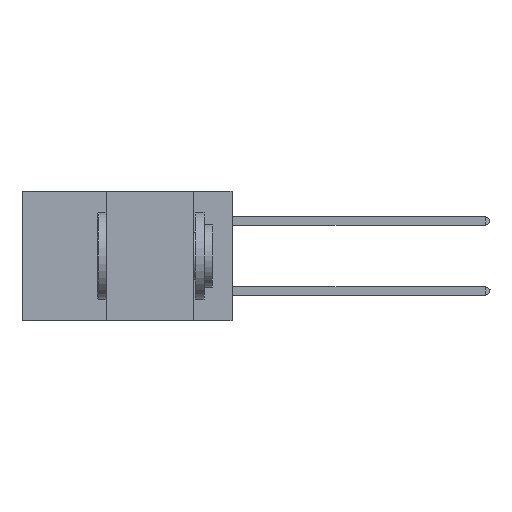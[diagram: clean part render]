
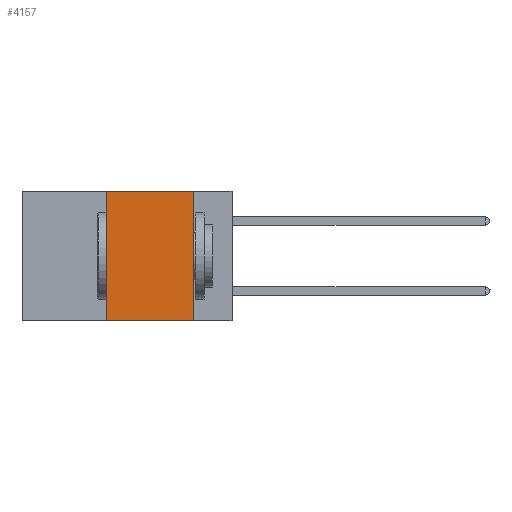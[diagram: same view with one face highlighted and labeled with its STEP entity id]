
A CAD part, left-side view. The second image highlights one B-rep face of the part: STEP entity #4157.
In plain terms, the highlighted planar face has unit normal (-1, 0, 0).
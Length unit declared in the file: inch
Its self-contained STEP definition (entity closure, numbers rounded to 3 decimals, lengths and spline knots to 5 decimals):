
#3628 = DIRECTION ( 'NONE',  ( 0., 0., 1. ) ) ;
#4157 = ADVANCED_FACE ( 'NONE', ( #16327 ), #21606, .F. ) ;
#4682 = LINE ( 'NONE', #5453, #26559 ) ;
#4757 = DIRECTION ( 'NONE',  ( 1., 0., 0. ) ) ;
#4849 = DIRECTION ( 'NONE',  ( 0., 0., -1. ) ) ;
#5453 = CARTESIAN_POINT ( 'NONE',  ( 0., 0.6, 0. ) ) ;
#6154 = VERTEX_POINT ( 'NONE', #26506 ) ;
#6286 = EDGE_CURVE ( 'NONE', #26279, #6154, #26335, .T. ) ;
#7574 = VERTEX_POINT ( 'NONE', #19311 ) ;
#7742 = AXIS2_PLACEMENT_3D ( 'NONE', #25572, #4757, #4849 ) ;
#14804 = EDGE_CURVE ( 'NONE', #7574, #6154, #24795, .T. ) ;
#15245 = LINE ( 'NONE', #22552, #20826 ) ;
#15635 = EDGE_CURVE ( 'NONE', #26279, #20886, #15245, .T. ) ;
#16327 = FACE_OUTER_BOUND ( 'NONE', #17850, .T. ) ;
#16593 = DIRECTION ( 'NONE',  ( 0., -1., 0. ) ) ;
#16954 = ORIENTED_EDGE ( 'NONE', *, *, #26620, .F. ) ;
#17660 = CARTESIAN_POINT ( 'NONE',  ( 0., 0.36, 0. ) ) ;
#17850 = EDGE_LOOP ( 'NONE', ( #20577, #16954, #18243, #25612 ) ) ;
#17911 = DIRECTION ( 'NONE',  ( 0., -1., 0. ) ) ;
#18243 = ORIENTED_EDGE ( 'NONE', *, *, #15635, .F. ) ;
#19311 = CARTESIAN_POINT ( 'NONE',  ( 0., 0.11, 0. ) ) ;
#19499 = DIRECTION ( 'NONE',  ( 0., 0., -1. ) ) ;
#20577 = ORIENTED_EDGE ( 'NONE', *, *, #14804, .F. ) ;
#20826 = VECTOR ( 'NONE', #3628, 39.37008 ) ;
#20880 = VECTOR ( 'NONE', #19499, 39.37008 ) ;
#20886 = VERTEX_POINT ( 'NONE', #17660 ) ;
#21134 = VECTOR ( 'NONE', #16593, 39.37008 ) ;
#21606 = PLANE ( 'NONE',  #7742 ) ;
#22552 = CARTESIAN_POINT ( 'NONE',  ( 0., 0.36, 0. ) ) ;
#23507 = CARTESIAN_POINT ( 'NONE',  ( 0., 0.6, -0.37 ) ) ;
#23869 = CARTESIAN_POINT ( 'NONE',  ( 0., 0.11, 0. ) ) ;
#24795 = LINE ( 'NONE', #23869, #20880 ) ;
#25349 = CARTESIAN_POINT ( 'NONE',  ( 0., 0.36, -0.37 ) ) ;
#25572 = CARTESIAN_POINT ( 'NONE',  ( 0., 0.6, 0. ) ) ;
#25612 = ORIENTED_EDGE ( 'NONE', *, *, #6286, .T. ) ;
#26279 = VERTEX_POINT ( 'NONE', #25349 ) ;
#26335 = LINE ( 'NONE', #23507, #21134 ) ;
#26506 = CARTESIAN_POINT ( 'NONE',  ( 0., 0.11, -0.37 ) ) ;
#26559 = VECTOR ( 'NONE', #17911, 39.37008 ) ;
#26620 = EDGE_CURVE ( 'NONE', #20886, #7574, #4682, .T. ) ;
